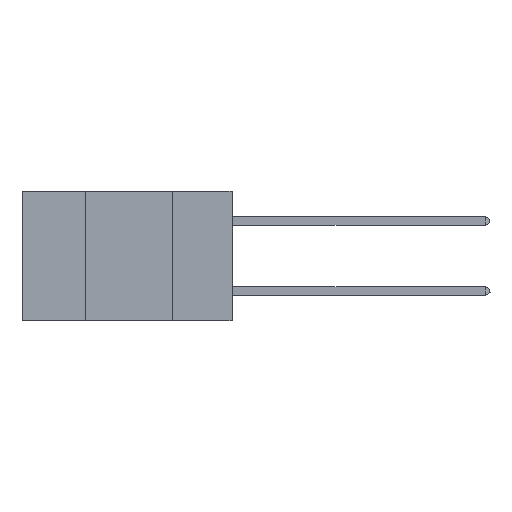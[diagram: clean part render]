
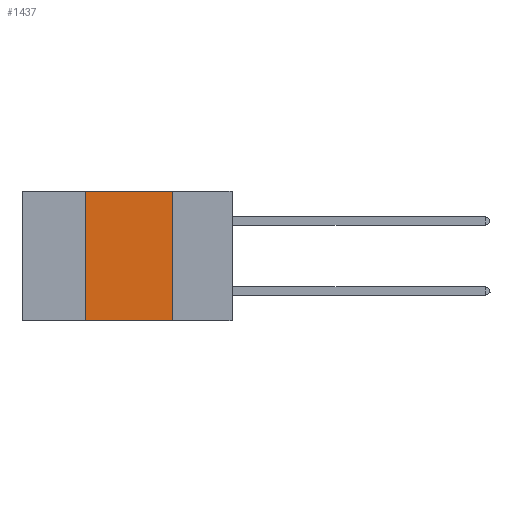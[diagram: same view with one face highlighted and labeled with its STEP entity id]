
A CAD part, left-side view. The second image highlights one B-rep face of the part: STEP entity #1437.
In plain terms, the highlighted planar face has unit normal (-1, 0, 0).
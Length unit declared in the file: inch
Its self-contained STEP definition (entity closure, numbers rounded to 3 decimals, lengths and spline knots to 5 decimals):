
#343 = PLANE ( 'NONE',  #2596 ) ;
#453 = EDGE_CURVE ( 'NONE', #14018, #9392, #6090, .T. ) ;
#1027 = DIRECTION ( 'NONE',  ( 0., -1., 0. ) ) ;
#1070 = CARTESIAN_POINT ( 'NONE',  ( 0., 0.6, -0.37 ) ) ;
#1249 = ORIENTED_EDGE ( 'NONE', *, *, #453, .F. ) ;
#1437 = ADVANCED_FACE ( 'NONE', ( #5166 ), #343, .F. ) ;
#1649 = DIRECTION ( 'NONE',  ( 0., 0., -1. ) ) ;
#1749 = ORIENTED_EDGE ( 'NONE', *, *, #5507, .T. ) ;
#2235 = DIRECTION ( 'NONE',  ( 0., -1., 0. ) ) ;
#2375 = CARTESIAN_POINT ( 'NONE',  ( 0., 0.42, 0. ) ) ;
#2596 = AXIS2_PLACEMENT_3D ( 'NONE', #10658, #8384, #5009 ) ;
#4038 = VECTOR ( 'NONE', #4515, 39.37008 ) ;
#4042 = EDGE_CURVE ( 'NONE', #11247, #14018, #4926, .T. ) ;
#4489 = EDGE_CURVE ( 'NONE', #9392, #9991, #6866, .T. ) ;
#4515 = DIRECTION ( 'NONE',  ( 0., 0., 1. ) ) ;
#4926 = LINE ( 'NONE', #6796, #4038 ) ;
#5009 = DIRECTION ( 'NONE',  ( 0., 0., -1. ) ) ;
#5166 = FACE_OUTER_BOUND ( 'NONE', #9092, .T. ) ;
#5280 = ORIENTED_EDGE ( 'NONE', *, *, #4042, .F. ) ;
#5507 = EDGE_CURVE ( 'NONE', #11247, #9991, #9716, .T. ) ;
#6090 = LINE ( 'NONE', #9895, #9087 ) ;
#6307 = ORIENTED_EDGE ( 'NONE', *, *, #4489, .F. ) ;
#6796 = CARTESIAN_POINT ( 'NONE',  ( 0., 0.42, 0. ) ) ;
#6866 = LINE ( 'NONE', #7156, #7225 ) ;
#7156 = CARTESIAN_POINT ( 'NONE',  ( 0., 0.17, 0. ) ) ;
#7225 = VECTOR ( 'NONE', #1649, 39.37008 ) ;
#8305 = VECTOR ( 'NONE', #2235, 39.37008 ) ;
#8384 = DIRECTION ( 'NONE',  ( 1., 0., 0. ) ) ;
#8501 = CARTESIAN_POINT ( 'NONE',  ( 0., 0.17, -0.37 ) ) ;
#8554 = CARTESIAN_POINT ( 'NONE',  ( 0., 0.17, 0. ) ) ;
#9087 = VECTOR ( 'NONE', #1027, 39.37008 ) ;
#9092 = EDGE_LOOP ( 'NONE', ( #6307, #1249, #5280, #1749 ) ) ;
#9392 = VERTEX_POINT ( 'NONE', #8554 ) ;
#9716 = LINE ( 'NONE', #1070, #8305 ) ;
#9895 = CARTESIAN_POINT ( 'NONE',  ( 0., 0.6, 0. ) ) ;
#9991 = VERTEX_POINT ( 'NONE', #8501 ) ;
#10658 = CARTESIAN_POINT ( 'NONE',  ( 0., 0.6, 0. ) ) ;
#11247 = VERTEX_POINT ( 'NONE', #11325 ) ;
#11325 = CARTESIAN_POINT ( 'NONE',  ( 0., 0.42, -0.37 ) ) ;
#14018 = VERTEX_POINT ( 'NONE', #2375 ) ;
